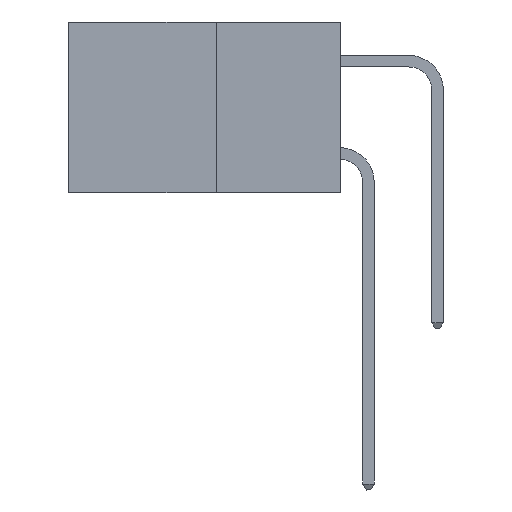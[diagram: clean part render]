
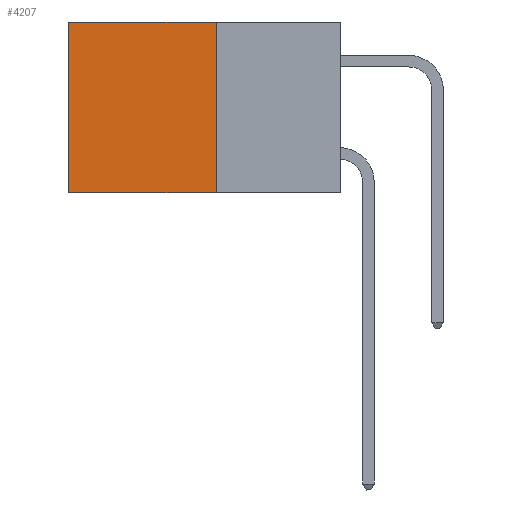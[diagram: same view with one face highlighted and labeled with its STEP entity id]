
A CAD part, left-side view. The second image highlights one B-rep face of the part: STEP entity #4207.
In plain terms, the highlighted planar face has unit normal (-1, 0, 0).
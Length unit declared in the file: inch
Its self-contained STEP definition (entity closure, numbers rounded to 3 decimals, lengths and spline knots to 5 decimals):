
#321 = EDGE_CURVE ( 'NONE', #4461, #9491, #2151, .T. ) ;
#747 = EDGE_CURVE ( 'NONE', #4461, #2294, #7151, .T. ) ;
#1648 = EDGE_LOOP ( 'NONE', ( #8819, #8685, #4256, #6748 ) ) ;
#1916 = CARTESIAN_POINT ( 'NONE',  ( 0.277, 0.27, -0.37 ) ) ;
#2042 = LINE ( 'NONE', #2973, #6255 ) ;
#2151 = LINE ( 'NONE', #1916, #11114 ) ;
#2294 = VERTEX_POINT ( 'NONE', #11394 ) ;
#2973 = CARTESIAN_POINT ( 'NONE',  ( 0.277, 0.59, -0.37 ) ) ;
#3290 = EDGE_CURVE ( 'NONE', #9491, #6723, #11629, .T. ) ;
#4207 = ADVANCED_FACE ( 'NONE', ( #5538 ), #9576, .F. ) ;
#4256 = ORIENTED_EDGE ( 'NONE', *, *, #321, .F. ) ;
#4376 = CARTESIAN_POINT ( 'NONE',  ( 0.277, 0.27, -0.37 ) ) ;
#4461 = VERTEX_POINT ( 'NONE', #10598 ) ;
#5265 = DIRECTION ( 'NONE',  ( 0., 0., -1. ) ) ;
#5538 = FACE_OUTER_BOUND ( 'NONE', #1648, .T. ) ;
#5695 = CARTESIAN_POINT ( 'NONE',  ( 0.277, 0.27, 0. ) ) ;
#6255 = VECTOR ( 'NONE', #6420, 39.37008 ) ;
#6420 = DIRECTION ( 'NONE',  ( 0., 0., -1. ) ) ;
#6723 = VERTEX_POINT ( 'NONE', #7234 ) ;
#6748 = ORIENTED_EDGE ( 'NONE', *, *, #747, .T. ) ;
#6902 = AXIS2_PLACEMENT_3D ( 'NONE', #4376, #10392, #5265 ) ;
#7151 = LINE ( 'NONE', #5695, #11098 ) ;
#7234 = CARTESIAN_POINT ( 'NONE',  ( 0.277, 0.59, -0.37 ) ) ;
#7649 = EDGE_CURVE ( 'NONE', #2294, #6723, #2042, .T. ) ;
#8211 = DIRECTION ( 'NONE',  ( 0., 0., -1. ) ) ;
#8685 = ORIENTED_EDGE ( 'NONE', *, *, #3290, .F. ) ;
#8819 = ORIENTED_EDGE ( 'NONE', *, *, #7649, .T. ) ;
#9491 = VERTEX_POINT ( 'NONE', #10648 ) ;
#9576 = PLANE ( 'NONE',  #6902 ) ;
#10083 = CARTESIAN_POINT ( 'NONE',  ( 0.277, 0.27, -0.37 ) ) ;
#10119 = DIRECTION ( 'NONE',  ( 0., 1., 0. ) ) ;
#10392 = DIRECTION ( 'NONE',  ( 1., 0., 0. ) ) ;
#10598 = CARTESIAN_POINT ( 'NONE',  ( 0.277, 0.27, 0. ) ) ;
#10648 = CARTESIAN_POINT ( 'NONE',  ( 0.277, 0.27, -0.37 ) ) ;
#11098 = VECTOR ( 'NONE', #11371, 39.37008 ) ;
#11114 = VECTOR ( 'NONE', #8211, 39.37008 ) ;
#11348 = VECTOR ( 'NONE', #10119, 39.37008 ) ;
#11371 = DIRECTION ( 'NONE',  ( 0., 1., 0. ) ) ;
#11394 = CARTESIAN_POINT ( 'NONE',  ( 0.277, 0.59, 0. ) ) ;
#11629 = LINE ( 'NONE', #10083, #11348 ) ;
